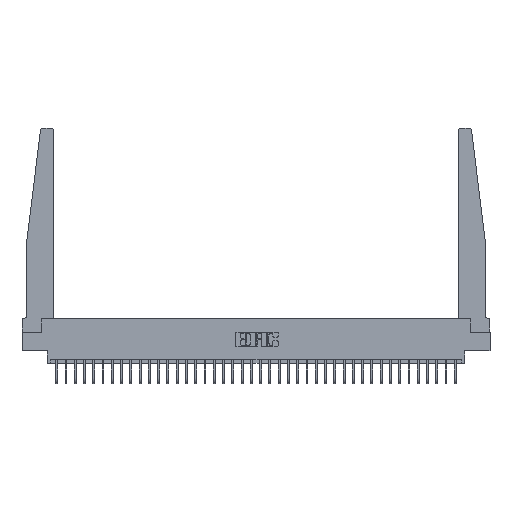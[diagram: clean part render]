
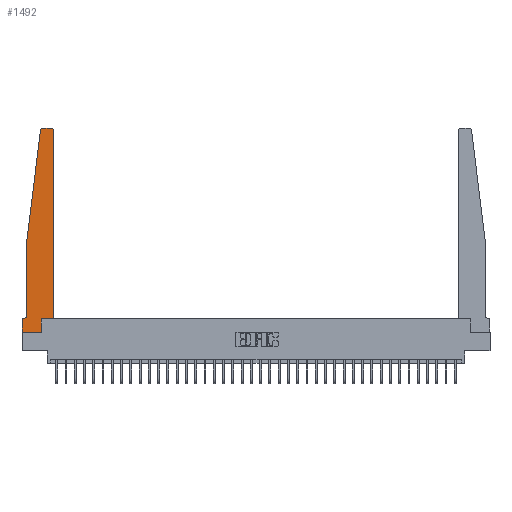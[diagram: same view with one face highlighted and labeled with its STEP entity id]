
A CAD part, top view. The second image highlights one B-rep face of the part: STEP entity #1492.
In plain terms, the highlighted planar face has unit normal (0, 0, 1).
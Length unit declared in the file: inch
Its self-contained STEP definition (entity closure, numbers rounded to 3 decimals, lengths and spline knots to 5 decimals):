
#115 = VERTEX_POINT ( 'NONE', #10801 ) ;
#740 = ORIENTED_EDGE ( 'NONE', *, *, #28321, .T. ) ;
#852 = LINE ( 'NONE', #5259, #17069 ) ;
#1239 = VECTOR ( 'NONE', #10950, 39.37008 ) ;
#1492 = ADVANCED_FACE ( 'NONE', ( #28782 ), #5918, .T. ) ;
#1535 = CARTESIAN_POINT ( 'NONE',  ( 0.2605, 0.18, 0.37 ) ) ;
#1574 = CARTESIAN_POINT ( 'NONE',  ( 0., 0., 0.37 ) ) ;
#1710 = EDGE_CURVE ( 'NONE', #15095, #25689, #23355, .T. ) ;
#1829 = LINE ( 'NONE', #4116, #18496 ) ;
#2000 = DIRECTION ( 'NONE',  ( -0.122, -0.992, 0. ) ) ;
#2164 = DIRECTION ( 'NONE',  ( -1., 0., 0. ) ) ;
#2984 = DIRECTION ( 'NONE',  ( -1., 0., 0. ) ) ;
#3295 = DIRECTION ( 'NONE',  ( 0., 0., 1. ) ) ;
#3700 = CARTESIAN_POINT ( 'NONE',  ( 0.395, 2.75, 0.37 ) ) ;
#3771 = VECTOR ( 'NONE', #31940, 39.37008 ) ;
#4077 = CARTESIAN_POINT ( 'NONE',  ( 0.425, 2.72, 0.37 ) ) ;
#4116 = CARTESIAN_POINT ( 'NONE',  ( 0.065, 1.25, 0.37 ) ) ;
#4801 = LINE ( 'NONE', #11891, #20060 ) ;
#5259 = CARTESIAN_POINT ( 'NONE',  ( 0.25, 2.75, 0.37 ) ) ;
#5585 = DIRECTION ( 'NONE',  ( 1., 0., 0. ) ) ;
#5851 = CIRCLE ( 'NONE', #20557, 0.03 ) ;
#5918 = PLANE ( 'NONE',  #10621 ) ;
#6013 = DIRECTION ( 'NONE',  ( 0., -1., 0. ) ) ;
#6243 = DIRECTION ( 'NONE',  ( 1., 0., 0. ) ) ;
#7362 = VECTOR ( 'NONE', #2164, 39.37008 ) ;
#7490 = ORIENTED_EDGE ( 'NONE', *, *, #16145, .T. ) ;
#7927 = VERTEX_POINT ( 'NONE', #4077 ) ;
#9060 = CARTESIAN_POINT ( 'NONE',  ( 0.065, 0.2375, 0.37 ) ) ;
#10033 = VERTEX_POINT ( 'NONE', #10112 ) ;
#10112 = CARTESIAN_POINT ( 'NONE',  ( 0., 0.1875, 0.37 ) ) ;
#10323 = ORIENTED_EDGE ( 'NONE', *, *, #26116, .T. ) ;
#10365 = ORIENTED_EDGE ( 'NONE', *, *, #30614, .T. ) ;
#10621 = AXIS2_PLACEMENT_3D ( 'NONE', #23701, #15804, #6243 ) ;
#10801 = CARTESIAN_POINT ( 'NONE',  ( 0.2605, 0., 0.37 ) ) ;
#10950 = DIRECTION ( 'NONE',  ( 0., -1., 0. ) ) ;
#11018 = EDGE_CURVE ( 'NONE', #18131, #12713, #1829, .T. ) ;
#11076 = EDGE_CURVE ( 'NONE', #26942, #115, #32037, .T. ) ;
#11454 = LINE ( 'NONE', #28549, #30575 ) ;
#11891 = CARTESIAN_POINT ( 'NONE',  ( 0.425, 0.18, 0.37 ) ) ;
#11901 = CARTESIAN_POINT ( 'NONE',  ( 0.425, 0.18, 0.37 ) ) ;
#12094 = DIRECTION ( 'NONE',  ( 0., 1., 0. ) ) ;
#12657 = DIRECTION ( 'NONE',  ( 0., 0., -1. ) ) ;
#12713 = VERTEX_POINT ( 'NONE', #25081 ) ;
#12984 = CARTESIAN_POINT ( 'NONE',  ( 0.015, 0.2375, 0.37 ) ) ;
#13007 = CARTESIAN_POINT ( 'NONE',  ( 0.27653, 2.72, 0.37 ) ) ;
#13171 = EDGE_CURVE ( 'NONE', #22088, #21491, #15182, .T. ) ;
#13325 = EDGE_LOOP ( 'NONE', ( #10365, #15321, #31174, #740, #24379, #10323, #7490, #26016, #24577, #29874, #30701, #26537 ) ) ;
#13754 = CARTESIAN_POINT ( 'NONE',  ( 0.395, 2.72, 0.37 ) ) ;
#14311 = AXIS2_PLACEMENT_3D ( 'NONE', #13007, #3295, #5585 ) ;
#14416 = EDGE_CURVE ( 'NONE', #115, #22088, #19830, .T. ) ;
#14639 = DIRECTION ( 'NONE',  ( 1., 0., 0. ) ) ;
#14783 = EDGE_CURVE ( 'NONE', #7927, #25720, #5851, .T. ) ;
#15095 = VERTEX_POINT ( 'NONE', #9060 ) ;
#15182 = LINE ( 'NONE', #11901, #3771 ) ;
#15321 = ORIENTED_EDGE ( 'NONE', *, *, #15383, .T. ) ;
#15383 = EDGE_CURVE ( 'NONE', #18340, #18131, #23233, .T. ) ;
#15804 = DIRECTION ( 'NONE',  ( 0., 0., 1. ) ) ;
#16145 = EDGE_CURVE ( 'NONE', #10033, #26942, #28368, .T. ) ;
#16531 = DIRECTION ( 'NONE',  ( 1., 0., 0. ) ) ;
#16947 = CARTESIAN_POINT ( 'NONE',  ( 0., 0., 0.37 ) ) ;
#17069 = VECTOR ( 'NONE', #2984, 39.37008 ) ;
#17127 = LINE ( 'NONE', #24650, #7362 ) ;
#17642 = VECTOR ( 'NONE', #14639, 39.37008 ) ;
#17757 = DIRECTION ( 'NONE',  ( -1., 0., 0. ) ) ;
#18131 = VERTEX_POINT ( 'NONE', #30981 ) ;
#18340 = VERTEX_POINT ( 'NONE', #29802 ) ;
#18496 = VECTOR ( 'NONE', #2000, 39.37008 ) ;
#19830 = LINE ( 'NONE', #25244, #28443 ) ;
#20060 = VECTOR ( 'NONE', #24859, 39.37008 ) ;
#20557 = AXIS2_PLACEMENT_3D ( 'NONE', #13754, #21784, #16531 ) ;
#21402 = CARTESIAN_POINT ( 'NONE',  ( 0.425, 0.18, 0.37 ) ) ;
#21491 = VERTEX_POINT ( 'NONE', #21402 ) ;
#21784 = DIRECTION ( 'NONE',  ( 0., 0., 1. ) ) ;
#21788 = CARTESIAN_POINT ( 'NONE',  ( 0.015, 0.1875, 0.37 ) ) ;
#22088 = VERTEX_POINT ( 'NONE', #1535 ) ;
#23233 = CIRCLE ( 'NONE', #14311, 0.03 ) ;
#23355 = CIRCLE ( 'NONE', #31734, 0.05 ) ;
#23701 = CARTESIAN_POINT ( 'NONE',  ( 0., 0.1875, 0.37 ) ) ;
#24379 = ORIENTED_EDGE ( 'NONE', *, *, #1710, .T. ) ;
#24577 = ORIENTED_EDGE ( 'NONE', *, *, #14416, .T. ) ;
#24650 = CARTESIAN_POINT ( 'NONE',  ( 0.065, 0.1875, 0.37 ) ) ;
#24859 = DIRECTION ( 'NONE',  ( 0., 1., 0. ) ) ;
#25081 = CARTESIAN_POINT ( 'NONE',  ( 0.065, 1.25, 0.37 ) ) ;
#25244 = CARTESIAN_POINT ( 'NONE',  ( 0.2605, 0.18, 0.37 ) ) ;
#25689 = VERTEX_POINT ( 'NONE', #21788 ) ;
#25720 = VERTEX_POINT ( 'NONE', #3700 ) ;
#26016 = ORIENTED_EDGE ( 'NONE', *, *, #11076, .T. ) ;
#26116 = EDGE_CURVE ( 'NONE', #25689, #10033, #17127, .T. ) ;
#26537 = ORIENTED_EDGE ( 'NONE', *, *, #14783, .T. ) ;
#26942 = VERTEX_POINT ( 'NONE', #1574 ) ;
#27060 = EDGE_CURVE ( 'NONE', #21491, #7927, #4801, .T. ) ;
#28321 = EDGE_CURVE ( 'NONE', #12713, #15095, #11454, .T. ) ;
#28368 = LINE ( 'NONE', #28535, #1239 ) ;
#28443 = VECTOR ( 'NONE', #12094, 39.37008 ) ;
#28535 = CARTESIAN_POINT ( 'NONE',  ( 0., 0., 0.37 ) ) ;
#28549 = CARTESIAN_POINT ( 'NONE',  ( 0.065, 1.25, 0.37 ) ) ;
#28782 = FACE_OUTER_BOUND ( 'NONE', #13325, .T. ) ;
#29802 = CARTESIAN_POINT ( 'NONE',  ( 0.27653, 2.75, 0.37 ) ) ;
#29874 = ORIENTED_EDGE ( 'NONE', *, *, #13171, .T. ) ;
#30575 = VECTOR ( 'NONE', #6013, 39.37008 ) ;
#30614 = EDGE_CURVE ( 'NONE', #25720, #18340, #852, .T. ) ;
#30701 = ORIENTED_EDGE ( 'NONE', *, *, #27060, .T. ) ;
#30981 = CARTESIAN_POINT ( 'NONE',  ( 0.24675, 2.72367, 0.37 ) ) ;
#31174 = ORIENTED_EDGE ( 'NONE', *, *, #11018, .T. ) ;
#31734 = AXIS2_PLACEMENT_3D ( 'NONE', #12984, #12657, #17757 ) ;
#31940 = DIRECTION ( 'NONE',  ( 1., 0., 0. ) ) ;
#32037 = LINE ( 'NONE', #16947, #17642 ) ;
